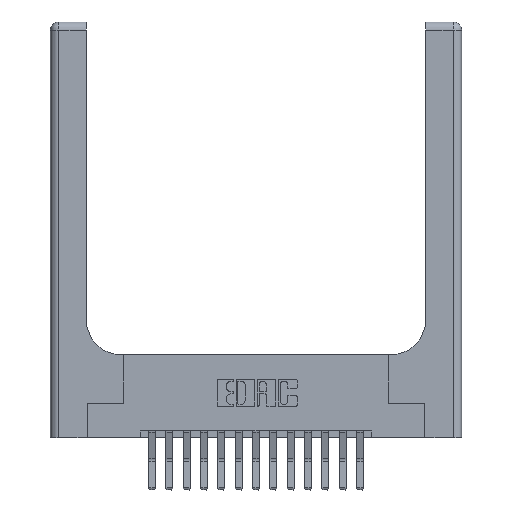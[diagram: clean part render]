
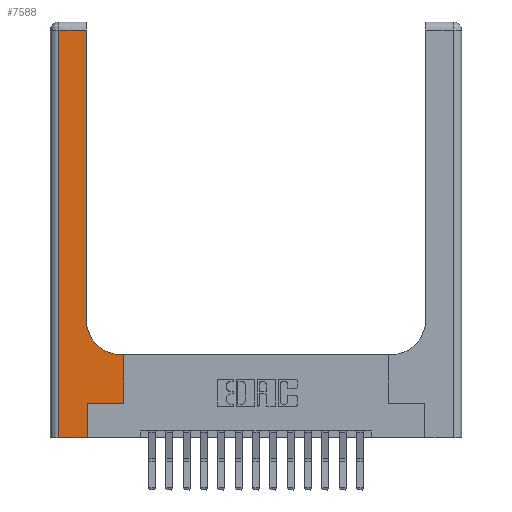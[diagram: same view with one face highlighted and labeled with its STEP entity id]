
A CAD part, top view. The second image highlights one B-rep face of the part: STEP entity #7588.
In plain terms, the highlighted planar face has unit normal (0, 0, 1).
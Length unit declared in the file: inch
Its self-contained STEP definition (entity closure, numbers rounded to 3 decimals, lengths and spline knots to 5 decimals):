
#184 = DIRECTION ( 'NONE',  ( -1., 0., 0. ) ) ;
#1119 = ORIENTED_EDGE ( 'NONE', *, *, #16134, .T. ) ;
#1301 = VERTEX_POINT ( 'NONE', #1933 ) ;
#1657 = LINE ( 'NONE', #4677, #16178 ) ;
#1735 = ORIENTED_EDGE ( 'NONE', *, *, #7123, .T. ) ;
#1831 = ORIENTED_EDGE ( 'NONE', *, *, #7333, .T. ) ;
#1933 = CARTESIAN_POINT ( 'NONE',  ( 0.528, 0.25, 0.37 ) ) ;
#2244 = CARTESIAN_POINT ( 'NONE',  ( 0.265, 0., 0.37 ) ) ;
#2350 = DIRECTION ( 'NONE',  ( 0., -1., 0. ) ) ;
#2378 = LINE ( 'NONE', #16385, #4161 ) ;
#3249 = CIRCLE ( 'NONE', #4717, 0.25 ) ;
#3279 = VECTOR ( 'NONE', #184, 39.37008 ) ;
#3591 = PLANE ( 'NONE',  #14643 ) ;
#3970 = DIRECTION ( 'NONE',  ( 0., 0., -1. ) ) ;
#4055 = VERTEX_POINT ( 'NONE', #9806 ) ;
#4161 = VECTOR ( 'NONE', #7834, 39.37008 ) ;
#4302 = CARTESIAN_POINT ( 'NONE',  ( 0.51, 0.6, 0.37 ) ) ;
#4531 = CARTESIAN_POINT ( 'NONE',  ( 0.06, 0., 0.37 ) ) ;
#4677 = CARTESIAN_POINT ( 'NONE',  ( 0.265, 0.25, 0.37 ) ) ;
#4717 = AXIS2_PLACEMENT_3D ( 'NONE', #6508, #3970, #6592 ) ;
#5302 = VECTOR ( 'NONE', #11529, 39.37008 ) ;
#5426 = CARTESIAN_POINT ( 'NONE',  ( 0.26, 0.85, 0.37 ) ) ;
#5922 = EDGE_CURVE ( 'NONE', #14012, #11722, #3249, .T. ) ;
#6308 = FACE_OUTER_BOUND ( 'NONE', #12845, .T. ) ;
#6331 = DIRECTION ( 'NONE',  ( 1., 0., 0. ) ) ;
#6436 = CARTESIAN_POINT ( 'NONE',  ( 0.06, 3., 0.37 ) ) ;
#6508 = CARTESIAN_POINT ( 'NONE',  ( 0.51, 0.85, 0.37 ) ) ;
#6592 = DIRECTION ( 'NONE',  ( 1., 0., 0. ) ) ;
#6630 = EDGE_CURVE ( 'NONE', #4055, #9044, #13221, .T. ) ;
#7123 = EDGE_CURVE ( 'NONE', #9044, #14667, #14671, .T. ) ;
#7149 = EDGE_CURVE ( 'NONE', #9151, #14012, #7872, .T. ) ;
#7207 = DIRECTION ( 'NONE',  ( 1., 0., 0. ) ) ;
#7296 = VECTOR ( 'NONE', #2350, 39.37008 ) ;
#7333 = EDGE_CURVE ( 'NONE', #11722, #12578, #10173, .T. ) ;
#7588 = ADVANCED_FACE ( 'NONE', ( #6308 ), #3591, .F. ) ;
#7759 = DIRECTION ( 'NONE',  ( 0., 0., -1. ) ) ;
#7815 = EDGE_CURVE ( 'NONE', #12578, #4055, #17115, .T. ) ;
#7834 = DIRECTION ( 'NONE',  ( 0., 1., 0. ) ) ;
#7872 = LINE ( 'NONE', #10722, #15833 ) ;
#7993 = EDGE_CURVE ( 'NONE', #1301, #9151, #2378, .T. ) ;
#8055 = CARTESIAN_POINT ( 'NONE',  ( 0.528, 0.6, 0.37 ) ) ;
#8346 = ORIENTED_EDGE ( 'NONE', *, *, #5922, .T. ) ;
#8722 = LINE ( 'NONE', #12859, #14767 ) ;
#8753 = CARTESIAN_POINT ( 'NONE',  ( 0., 2.94, 0.37 ) ) ;
#9044 = VERTEX_POINT ( 'NONE', #4531 ) ;
#9128 = ORIENTED_EDGE ( 'NONE', *, *, #7149, .T. ) ;
#9151 = VERTEX_POINT ( 'NONE', #8055 ) ;
#9311 = ORIENTED_EDGE ( 'NONE', *, *, #6630, .T. ) ;
#9806 = CARTESIAN_POINT ( 'NONE',  ( 0.06, 2.94, 0.37 ) ) ;
#10173 = LINE ( 'NONE', #17048, #5302 ) ;
#10722 = CARTESIAN_POINT ( 'NONE',  ( 0.26, 0.6, 0.37 ) ) ;
#11039 = EDGE_CURVE ( 'NONE', #16444, #1301, #1657, .T. ) ;
#11479 = DIRECTION ( 'NONE',  ( 0., 1., 0. ) ) ;
#11529 = DIRECTION ( 'NONE',  ( 0., 1., 0. ) ) ;
#11722 = VERTEX_POINT ( 'NONE', #5426 ) ;
#12276 = VECTOR ( 'NONE', #6331, 39.37008 ) ;
#12578 = VERTEX_POINT ( 'NONE', #13161 ) ;
#12845 = EDGE_LOOP ( 'NONE', ( #1831, #17930, #9311, #1735, #1119, #15169, #16290, #9128, #8346 ) ) ;
#12859 = CARTESIAN_POINT ( 'NONE',  ( 0.265, 0., 0.37 ) ) ;
#13084 = CARTESIAN_POINT ( 'NONE',  ( 0.265, 0.25, 0.37 ) ) ;
#13161 = CARTESIAN_POINT ( 'NONE',  ( 0.26, 2.94, 0.37 ) ) ;
#13221 = LINE ( 'NONE', #6436, #7296 ) ;
#13361 = DIRECTION ( 'NONE',  ( -1., 0., 0. ) ) ;
#14012 = VERTEX_POINT ( 'NONE', #4302 ) ;
#14643 = AXIS2_PLACEMENT_3D ( 'NONE', #16141, #7759, #13361 ) ;
#14667 = VERTEX_POINT ( 'NONE', #2244 ) ;
#14671 = LINE ( 'NONE', #17526, #12276 ) ;
#14767 = VECTOR ( 'NONE', #11479, 39.37008 ) ;
#15169 = ORIENTED_EDGE ( 'NONE', *, *, #11039, .T. ) ;
#15833 = VECTOR ( 'NONE', #16339, 39.37008 ) ;
#16134 = EDGE_CURVE ( 'NONE', #14667, #16444, #8722, .T. ) ;
#16141 = CARTESIAN_POINT ( 'NONE',  ( 0., 3., 0.37 ) ) ;
#16178 = VECTOR ( 'NONE', #7207, 39.37008 ) ;
#16290 = ORIENTED_EDGE ( 'NONE', *, *, #7993, .T. ) ;
#16339 = DIRECTION ( 'NONE',  ( -1., 0., 0. ) ) ;
#16385 = CARTESIAN_POINT ( 'NONE',  ( 0.528, 0.25, 0.37 ) ) ;
#16444 = VERTEX_POINT ( 'NONE', #13084 ) ;
#17048 = CARTESIAN_POINT ( 'NONE',  ( 0.26, 3., 0.37 ) ) ;
#17115 = LINE ( 'NONE', #8753, #3279 ) ;
#17526 = CARTESIAN_POINT ( 'NONE',  ( 0., 0., 0.37 ) ) ;
#17930 = ORIENTED_EDGE ( 'NONE', *, *, #7815, .T. ) ;
